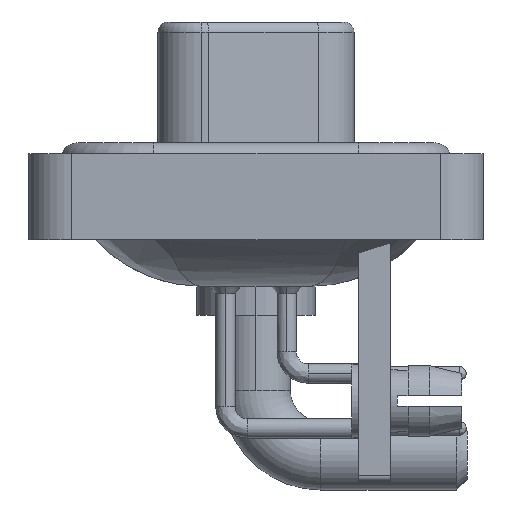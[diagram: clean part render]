
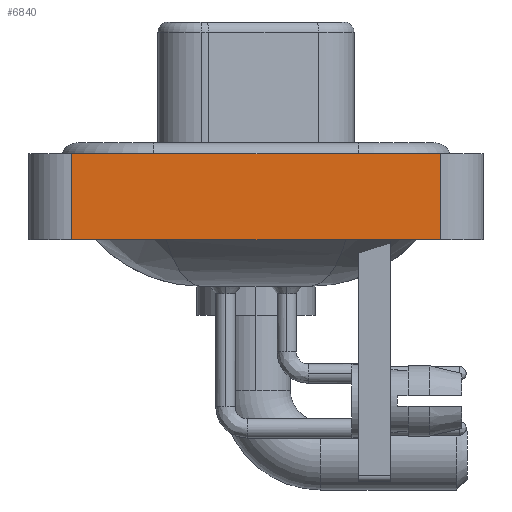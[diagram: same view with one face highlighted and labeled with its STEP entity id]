
A CAD part, left-side view. The second image highlights one B-rep face of the part: STEP entity #6840.
In plain terms, the highlighted planar face has unit normal (-1, 0, 0).
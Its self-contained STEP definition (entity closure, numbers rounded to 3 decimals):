
#342 = ORIENTED_EDGE ( 'NONE', *, *, #10360, .T. ) ;
#1291 = EDGE_CURVE ( 'NONE', #18866, #4032, #17252, .T. ) ;
#1349 = CARTESIAN_POINT ( 'NONE',  ( -7.25, -8.55, -3.6 ) ) ;
#2296 = VECTOR ( 'NONE', #17941, 1000. ) ;
#4032 = VERTEX_POINT ( 'NONE', #19225 ) ;
#5579 = CARTESIAN_POINT ( 'NONE',  ( -7.25, -8.55, -3.6 ) ) ;
#6177 = CARTESIAN_POINT ( 'NONE',  ( -7.25, 8.55, -3.6 ) ) ;
#6840 = ADVANCED_FACE ( 'NONE', ( #23928 ), #22255, .T. ) ;
#8112 = LINE ( 'NONE', #6177, #2296 ) ;
#8113 = EDGE_LOOP ( 'NONE', ( #342, #12834, #20652, #21688 ) ) ;
#8953 = CARTESIAN_POINT ( 'NONE',  ( -7.25, -8.55, -3.6 ) ) ;
#10360 = EDGE_CURVE ( 'NONE', #20945, #4032, #24989, .T. ) ;
#12369 = VECTOR ( 'NONE', #20941, 1000. ) ;
#12834 = ORIENTED_EDGE ( 'NONE', *, *, #1291, .F. ) ;
#13325 = AXIS2_PLACEMENT_3D ( 'NONE', #16161, #18319, #19735 ) ;
#13375 = DIRECTION ( 'NONE',  ( 0., 0., 1. ) ) ;
#14735 = EDGE_CURVE ( 'NONE', #22796, #20945, #18284, .T. ) ;
#16161 = CARTESIAN_POINT ( 'NONE',  ( -7.25, -8.55, -3.6 ) ) ;
#16483 = DIRECTION ( 'NONE',  ( 0., -1., 0. ) ) ;
#17252 = LINE ( 'NONE', #22848, #12369 ) ;
#17941 = DIRECTION ( 'NONE',  ( 0., 0., 1. ) ) ;
#18279 = VECTOR ( 'NONE', #16483, 1000. ) ;
#18284 = LINE ( 'NONE', #8953, #18279 ) ;
#18319 = DIRECTION ( 'NONE',  ( -1., 0., 0. ) ) ;
#18866 = VERTEX_POINT ( 'NONE', #18886 ) ;
#18886 = CARTESIAN_POINT ( 'NONE',  ( -7.25, 8.55, 0.4 ) ) ;
#19225 = CARTESIAN_POINT ( 'NONE',  ( -7.25, -8.55, 0.4 ) ) ;
#19735 = DIRECTION ( 'NONE',  ( 0., 0., 1. ) ) ;
#20292 = CARTESIAN_POINT ( 'NONE',  ( -7.25, 8.55, -3.6 ) ) ;
#20652 = ORIENTED_EDGE ( 'NONE', *, *, #21162, .F. ) ;
#20941 = DIRECTION ( 'NONE',  ( 0., -1., 0. ) ) ;
#20945 = VERTEX_POINT ( 'NONE', #1349 ) ;
#21162 = EDGE_CURVE ( 'NONE', #22796, #18866, #8112, .T. ) ;
#21688 = ORIENTED_EDGE ( 'NONE', *, *, #14735, .T. ) ;
#22255 = PLANE ( 'NONE',  #13325 ) ;
#22426 = VECTOR ( 'NONE', #13375, 1000. ) ;
#22796 = VERTEX_POINT ( 'NONE', #20292 ) ;
#22848 = CARTESIAN_POINT ( 'NONE',  ( -7.25, -8.55, 0.4 ) ) ;
#23928 = FACE_OUTER_BOUND ( 'NONE', #8113, .T. ) ;
#24989 = LINE ( 'NONE', #5579, #22426 ) ;
